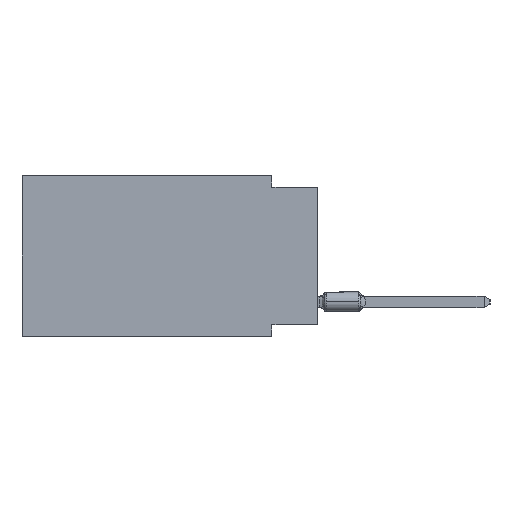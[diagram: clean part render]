
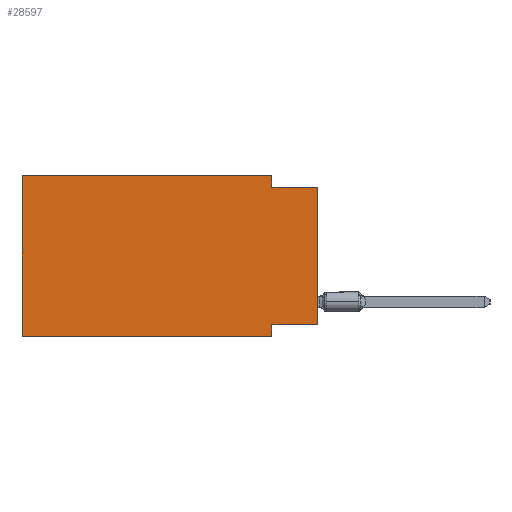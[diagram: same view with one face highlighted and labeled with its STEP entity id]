
A CAD part, left-side view. The second image highlights one B-rep face of the part: STEP entity #28597.
In plain terms, the highlighted planar face has unit normal (-1, 0, 0).
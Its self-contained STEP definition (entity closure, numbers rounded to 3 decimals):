
#909 = CARTESIAN_POINT ( 'NONE',  ( 0., 0., 0. ) ) ;
#999 = VECTOR ( 'NONE', #29394, 1000. ) ;
#1042 = EDGE_LOOP ( 'NONE', ( #31770, #12962, #3595, #27356, #14594, #12578, #16659, #21501 ) ) ;
#1197 = VERTEX_POINT ( 'NONE', #41688 ) ;
#2099 = DIRECTION ( 'NONE',  ( 0., 0., -1. ) ) ;
#2110 = LINE ( 'NONE', #28817, #7153 ) ;
#2284 = CARTESIAN_POINT ( 'NONE',  ( 0., 16.383, 0. ) ) ;
#3595 = ORIENTED_EDGE ( 'NONE', *, *, #27000, .F. ) ;
#4557 = VERTEX_POINT ( 'NONE', #7080 ) ;
#4855 = EDGE_CURVE ( 'NONE', #13508, #32679, #27232, .T. ) ;
#6054 = VECTOR ( 'NONE', #7461, 1000. ) ;
#6090 = FACE_OUTER_BOUND ( 'NONE', #1042, .T. ) ;
#6549 = PLANE ( 'NONE',  #37206 ) ;
#7080 = CARTESIAN_POINT ( 'NONE',  ( 0., 2.54, -8.89 ) ) ;
#7153 = VECTOR ( 'NONE', #22083, 1000. ) ;
#7461 = DIRECTION ( 'NONE',  ( 0., 0., 1. ) ) ;
#8233 = CARTESIAN_POINT ( 'NONE',  ( 0., 0., -0.635 ) ) ;
#8523 = VERTEX_POINT ( 'NONE', #18077 ) ;
#9076 = LINE ( 'NONE', #32905, #22401 ) ;
#11110 = CARTESIAN_POINT ( 'NONE',  ( 0., 0., -8.255 ) ) ;
#11166 = LINE ( 'NONE', #8233, #36446 ) ;
#11470 = DIRECTION ( 'NONE',  ( 0., 0., 1. ) ) ;
#12578 = ORIENTED_EDGE ( 'NONE', *, *, #24542, .T. ) ;
#12895 = DIRECTION ( 'NONE',  ( 0., 0., -1. ) ) ;
#12962 = ORIENTED_EDGE ( 'NONE', *, *, #18742, .F. ) ;
#13508 = VERTEX_POINT ( 'NONE', #31317 ) ;
#14591 = VECTOR ( 'NONE', #18198, 1000. ) ;
#14594 = ORIENTED_EDGE ( 'NONE', *, *, #4855, .F. ) ;
#16659 = ORIENTED_EDGE ( 'NONE', *, *, #34058, .F. ) ;
#16796 = VERTEX_POINT ( 'NONE', #11110 ) ;
#18077 = CARTESIAN_POINT ( 'NONE',  ( 0., 2.54, -8.255 ) ) ;
#18198 = DIRECTION ( 'NONE',  ( 0., -1., 0. ) ) ;
#18399 = LINE ( 'NONE', #909, #44195 ) ;
#18742 = EDGE_CURVE ( 'NONE', #19676, #26576, #11166, .T. ) ;
#19058 = CARTESIAN_POINT ( 'NONE',  ( 0., 0., -8.255 ) ) ;
#19676 = VERTEX_POINT ( 'NONE', #35609 ) ;
#21501 = ORIENTED_EDGE ( 'NONE', *, *, #37666, .F. ) ;
#22083 = DIRECTION ( 'NONE',  ( 0., -1., 0. ) ) ;
#22401 = VECTOR ( 'NONE', #12895, 1000. ) ;
#22418 = LINE ( 'NONE', #19058, #999 ) ;
#23609 = DIRECTION ( 'NONE',  ( 0., 0., -1. ) ) ;
#24239 = VECTOR ( 'NONE', #2099, 1000. ) ;
#24542 = EDGE_CURVE ( 'NONE', #13508, #4557, #38422, .T. ) ;
#24740 = CARTESIAN_POINT ( 'NONE',  ( 0., 16.383, 0. ) ) ;
#25295 = DIRECTION ( 'NONE',  ( 0., -1., 0. ) ) ;
#26576 = VERTEX_POINT ( 'NONE', #41760 ) ;
#27000 = EDGE_CURVE ( 'NONE', #1197, #19676, #28808, .T. ) ;
#27232 = LINE ( 'NONE', #24740, #6054 ) ;
#27356 = ORIENTED_EDGE ( 'NONE', *, *, #28129, .F. ) ;
#28129 = EDGE_CURVE ( 'NONE', #32679, #1197, #2110, .T. ) ;
#28597 = ADVANCED_FACE ( 'NONE', ( #6090 ), #6549, .F. ) ;
#28808 = LINE ( 'NONE', #42500, #24239 ) ;
#28817 = CARTESIAN_POINT ( 'NONE',  ( 0., 16.383, 0. ) ) ;
#29394 = DIRECTION ( 'NONE',  ( 0., 1., 0. ) ) ;
#31317 = CARTESIAN_POINT ( 'NONE',  ( 0., 16.383, -8.89 ) ) ;
#31470 = CARTESIAN_POINT ( 'NONE',  ( 0., 16.383, -8.89 ) ) ;
#31770 = ORIENTED_EDGE ( 'NONE', *, *, #40017, .T. ) ;
#32679 = VERTEX_POINT ( 'NONE', #38738 ) ;
#32905 = CARTESIAN_POINT ( 'NONE',  ( 0., 2.54, -8.89 ) ) ;
#34058 = EDGE_CURVE ( 'NONE', #8523, #4557, #9076, .T. ) ;
#35609 = CARTESIAN_POINT ( 'NONE',  ( 0., 2.54, -0.635 ) ) ;
#36418 = DIRECTION ( 'NONE',  ( 1., 0., 0. ) ) ;
#36446 = VECTOR ( 'NONE', #25295, 1000. ) ;
#37206 = AXIS2_PLACEMENT_3D ( 'NONE', #2284, #36418, #23609 ) ;
#37666 = EDGE_CURVE ( 'NONE', #16796, #8523, #22418, .T. ) ;
#38422 = LINE ( 'NONE', #31470, #14591 ) ;
#38738 = CARTESIAN_POINT ( 'NONE',  ( 0., 16.383, 0. ) ) ;
#40017 = EDGE_CURVE ( 'NONE', #16796, #26576, #18399, .T. ) ;
#41688 = CARTESIAN_POINT ( 'NONE',  ( 0., 2.54, 0. ) ) ;
#41760 = CARTESIAN_POINT ( 'NONE',  ( 0., 0., -0.635 ) ) ;
#42500 = CARTESIAN_POINT ( 'NONE',  ( 0., 2.54, 0. ) ) ;
#44195 = VECTOR ( 'NONE', #11470, 1000. ) ;
